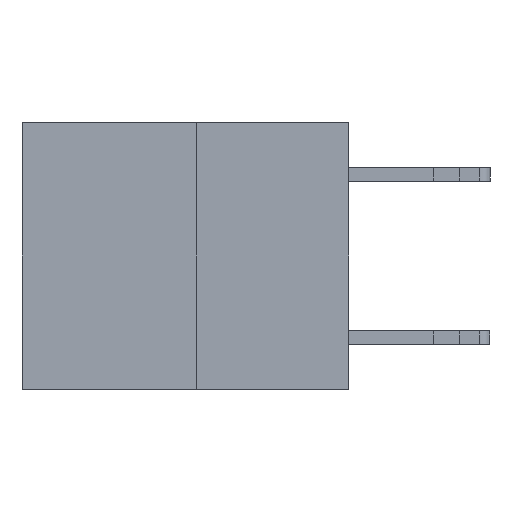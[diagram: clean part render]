
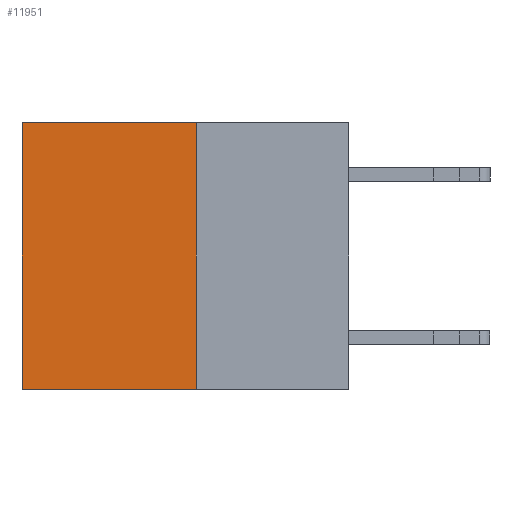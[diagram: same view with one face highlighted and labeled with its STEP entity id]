
A CAD part, left-side view. The second image highlights one B-rep face of the part: STEP entity #11951.
In plain terms, the highlighted planar face has unit normal (-1, 0, 0).
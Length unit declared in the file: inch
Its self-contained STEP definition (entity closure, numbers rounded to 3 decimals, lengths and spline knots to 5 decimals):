
#442 = VECTOR ( 'NONE', #8575, 39.37008 ) ;
#535 = CARTESIAN_POINT ( 'NONE',  ( 0.3165, 0.6, -0.49 ) ) ;
#1205 = CARTESIAN_POINT ( 'NONE',  ( 0.3165, 0.28, -0.49 ) ) ;
#2154 = EDGE_CURVE ( 'NONE', #9278, #11717, #10109, .T. ) ;
#2597 = ORIENTED_EDGE ( 'NONE', *, *, #12580, .F. ) ;
#4412 = LINE ( 'NONE', #18259, #17702 ) ;
#5293 = ORIENTED_EDGE ( 'NONE', *, *, #11033, .T. ) ;
#5468 = AXIS2_PLACEMENT_3D ( 'NONE', #1205, #7256, #19098 ) ;
#7256 = DIRECTION ( 'NONE',  ( 1., 0., 0. ) ) ;
#7283 = VECTOR ( 'NONE', #9561, 39.37008 ) ;
#8011 = CARTESIAN_POINT ( 'NONE',  ( 0.3165, 0.28, 0. ) ) ;
#8575 = DIRECTION ( 'NONE',  ( 0., 1., 0. ) ) ;
#8682 = CARTESIAN_POINT ( 'NONE',  ( 0.3165, 0.28, -0.49 ) ) ;
#9167 = DIRECTION ( 'NONE',  ( 0., 0., -1. ) ) ;
#9278 = VERTEX_POINT ( 'NONE', #16136 ) ;
#9561 = DIRECTION ( 'NONE',  ( 0., 0., -1. ) ) ;
#9929 = VERTEX_POINT ( 'NONE', #15199 ) ;
#9974 = LINE ( 'NONE', #8682, #16904 ) ;
#10109 = LINE ( 'NONE', #535, #7283 ) ;
#10287 = VERTEX_POINT ( 'NONE', #8011 ) ;
#10297 = CARTESIAN_POINT ( 'NONE',  ( 0.3165, 0.28, 0. ) ) ;
#11033 = EDGE_CURVE ( 'NONE', #10287, #9278, #14431, .T. ) ;
#11137 = ORIENTED_EDGE ( 'NONE', *, *, #13023, .F. ) ;
#11717 = VERTEX_POINT ( 'NONE', #13115 ) ;
#11951 = ADVANCED_FACE ( 'NONE', ( #18520 ), #19166, .F. ) ;
#12580 = EDGE_CURVE ( 'NONE', #9929, #11717, #9974, .T. ) ;
#12885 = ORIENTED_EDGE ( 'NONE', *, *, #2154, .T. ) ;
#13023 = EDGE_CURVE ( 'NONE', #10287, #9929, #4412, .T. ) ;
#13115 = CARTESIAN_POINT ( 'NONE',  ( 0.3165, 0.6, -0.49 ) ) ;
#13358 = DIRECTION ( 'NONE',  ( 0., 1., 0. ) ) ;
#14431 = LINE ( 'NONE', #10297, #442 ) ;
#15199 = CARTESIAN_POINT ( 'NONE',  ( 0.3165, 0.28, -0.49 ) ) ;
#16003 = EDGE_LOOP ( 'NONE', ( #12885, #2597, #11137, #5293 ) ) ;
#16136 = CARTESIAN_POINT ( 'NONE',  ( 0.3165, 0.6, 0. ) ) ;
#16904 = VECTOR ( 'NONE', #13358, 39.37008 ) ;
#17702 = VECTOR ( 'NONE', #9167, 39.37008 ) ;
#18259 = CARTESIAN_POINT ( 'NONE',  ( 0.3165, 0.28, -0.49 ) ) ;
#18520 = FACE_OUTER_BOUND ( 'NONE', #16003, .T. ) ;
#19098 = DIRECTION ( 'NONE',  ( 0., 0., -1. ) ) ;
#19166 = PLANE ( 'NONE',  #5468 ) ;
